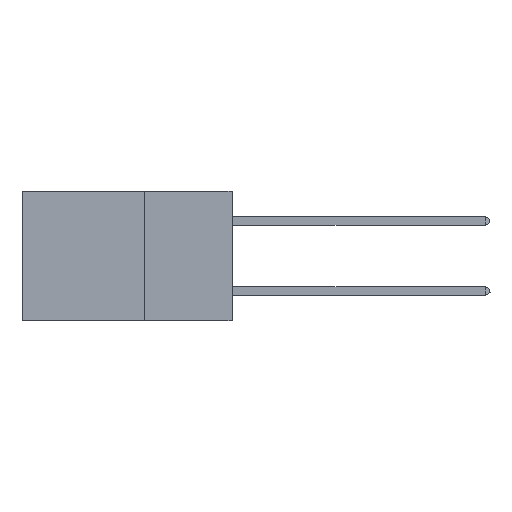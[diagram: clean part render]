
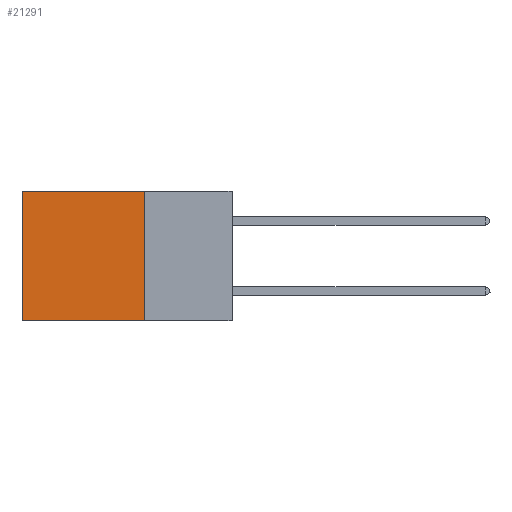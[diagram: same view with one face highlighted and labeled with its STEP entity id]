
A CAD part, left-side view. The second image highlights one B-rep face of the part: STEP entity #21291.
In plain terms, the highlighted planar face has unit normal (-1, 0, 0).
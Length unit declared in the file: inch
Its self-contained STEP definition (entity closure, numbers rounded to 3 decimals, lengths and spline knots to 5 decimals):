
#447 = LINE ( 'NONE', #20066, #28584 ) ;
#3681 = VECTOR ( 'NONE', #26134, 39.37008 ) ;
#3833 = EDGE_CURVE ( 'NONE', #6368, #26740, #21763, .T. ) ;
#4098 = DIRECTION ( 'NONE',  ( 0., 1., 0. ) ) ;
#4123 = LINE ( 'NONE', #8569, #26343 ) ;
#6092 = ORIENTED_EDGE ( 'NONE', *, *, #21246, .T. ) ;
#6368 = VERTEX_POINT ( 'NONE', #21616 ) ;
#6433 = DIRECTION ( 'NONE',  ( 1., 0., 0. ) ) ;
#6844 = VERTEX_POINT ( 'NONE', #26256 ) ;
#8569 = CARTESIAN_POINT ( 'NONE',  ( 0.2875, 0.25, -0.37 ) ) ;
#9388 = VECTOR ( 'NONE', #10658, 39.37008 ) ;
#9882 = CARTESIAN_POINT ( 'NONE',  ( 0.2875, 0.6, 0. ) ) ;
#10658 = DIRECTION ( 'NONE',  ( 0., 0., -1. ) ) ;
#12491 = AXIS2_PLACEMENT_3D ( 'NONE', #17594, #6433, #21946 ) ;
#13274 = DIRECTION ( 'NONE',  ( 0., 1., 0. ) ) ;
#15479 = ORIENTED_EDGE ( 'NONE', *, *, #24471, .F. ) ;
#15810 = ORIENTED_EDGE ( 'NONE', *, *, #26850, .T. ) ;
#16954 = EDGE_LOOP ( 'NONE', ( #15810, #15479, #27381, #6092 ) ) ;
#17594 = CARTESIAN_POINT ( 'NONE',  ( 0.2875, 0.25, 0. ) ) ;
#20066 = CARTESIAN_POINT ( 'NONE',  ( 0.2875, 0.25, 0. ) ) ;
#21246 = EDGE_CURVE ( 'NONE', #6368, #27409, #447, .T. ) ;
#21291 = ADVANCED_FACE ( 'NONE', ( #23029 ), #28656, .F. ) ;
#21616 = CARTESIAN_POINT ( 'NONE',  ( 0.2875, 0.25, 0. ) ) ;
#21763 = LINE ( 'NONE', #28275, #3681 ) ;
#21946 = DIRECTION ( 'NONE',  ( 0., 0., -1. ) ) ;
#23029 = FACE_OUTER_BOUND ( 'NONE', #16954, .T. ) ;
#23156 = CARTESIAN_POINT ( 'NONE',  ( 0.2875, 0.25, -0.37 ) ) ;
#23797 = CARTESIAN_POINT ( 'NONE',  ( 0.2875, 0.6, 0. ) ) ;
#24471 = EDGE_CURVE ( 'NONE', #26740, #6844, #4123, .T. ) ;
#26134 = DIRECTION ( 'NONE',  ( 0., 0., -1. ) ) ;
#26256 = CARTESIAN_POINT ( 'NONE',  ( 0.2875, 0.6, -0.37 ) ) ;
#26343 = VECTOR ( 'NONE', #13274, 39.37008 ) ;
#26740 = VERTEX_POINT ( 'NONE', #23156 ) ;
#26850 = EDGE_CURVE ( 'NONE', #27409, #6844, #28508, .T. ) ;
#27381 = ORIENTED_EDGE ( 'NONE', *, *, #3833, .F. ) ;
#27409 = VERTEX_POINT ( 'NONE', #9882 ) ;
#28275 = CARTESIAN_POINT ( 'NONE',  ( 0.2875, 0.25, 0. ) ) ;
#28508 = LINE ( 'NONE', #23797, #9388 ) ;
#28584 = VECTOR ( 'NONE', #4098, 39.37008 ) ;
#28656 = PLANE ( 'NONE',  #12491 ) ;
